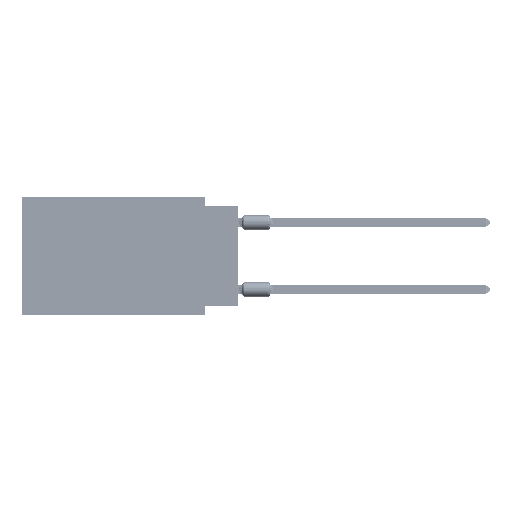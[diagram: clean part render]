
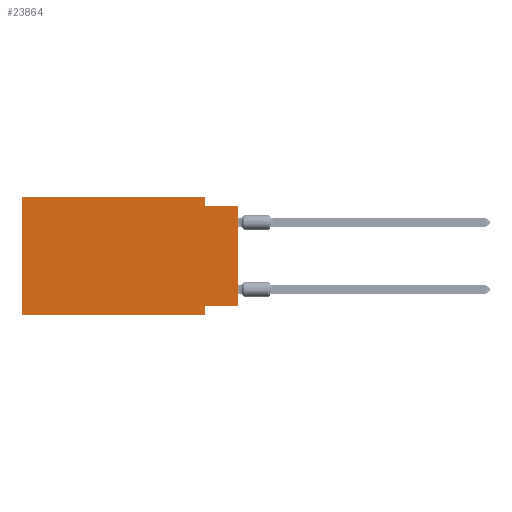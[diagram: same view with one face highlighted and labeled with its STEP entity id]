
A CAD part, left-side view. The second image highlights one B-rep face of the part: STEP entity #23864.
In plain terms, the highlighted planar face has unit normal (-1, 0, 0).
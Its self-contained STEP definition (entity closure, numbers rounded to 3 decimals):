
#1784 = DIRECTION ( 'NONE',  ( 0., -1., 0. ) ) ;
#3954 = ORIENTED_EDGE ( 'NONE', *, *, #64377, .T. ) ;
#4274 = EDGE_CURVE ( 'NONE', #51463, #29022, #56567, .T. ) ;
#5996 = CARTESIAN_POINT ( 'NONE',  ( 0., 2.54, 0. ) ) ;
#6498 = VERTEX_POINT ( 'NONE', #27731 ) ;
#7110 = CARTESIAN_POINT ( 'NONE',  ( 0., 16.383, 0. ) ) ;
#8645 = LINE ( 'NONE', #40354, #41786 ) ;
#8923 = CARTESIAN_POINT ( 'NONE',  ( 0., 0., -0.635 ) ) ;
#9326 = ORIENTED_EDGE ( 'NONE', *, *, #33145, .F. ) ;
#9361 = CARTESIAN_POINT ( 'NONE',  ( 0., 16.383, -8.89 ) ) ;
#11663 = ORIENTED_EDGE ( 'NONE', *, *, #61081, .F. ) ;
#13137 = DIRECTION ( 'NONE',  ( 0., 0., -1. ) ) ;
#14326 = DIRECTION ( 'NONE',  ( 0., 0., -1. ) ) ;
#15035 = DIRECTION ( 'NONE',  ( 0., -1., 0. ) ) ;
#16215 = EDGE_CURVE ( 'NONE', #34249, #54999, #58477, .T. ) ;
#17212 = VERTEX_POINT ( 'NONE', #51149 ) ;
#18328 = DIRECTION ( 'NONE',  ( 0., 0., -1. ) ) ;
#18995 = LINE ( 'NONE', #35566, #62263 ) ;
#19801 = DIRECTION ( 'NONE',  ( 0., 0., 1. ) ) ;
#22435 = CARTESIAN_POINT ( 'NONE',  ( 0., 2.54, -0.635 ) ) ;
#22471 = EDGE_LOOP ( 'NONE', ( #30737, #26094, #35533, #25696, #65704, #3954, #9326, #11663 ) ) ;
#22800 = VECTOR ( 'NONE', #19801, 1000. ) ;
#23864 = ADVANCED_FACE ( 'NONE', ( #63270 ), #43198, .F. ) ;
#24582 = EDGE_CURVE ( 'NONE', #6498, #34249, #60778, .T. ) ;
#25696 = ORIENTED_EDGE ( 'NONE', *, *, #16215, .F. ) ;
#26094 = ORIENTED_EDGE ( 'NONE', *, *, #4274, .F. ) ;
#27631 = VECTOR ( 'NONE', #57805, 1000. ) ;
#27731 = CARTESIAN_POINT ( 'NONE',  ( 0., 16.383, -8.89 ) ) ;
#29022 = VERTEX_POINT ( 'NONE', #8923 ) ;
#30737 = ORIENTED_EDGE ( 'NONE', *, *, #37418, .T. ) ;
#33145 = EDGE_CURVE ( 'NONE', #17212, #58253, #8645, .T. ) ;
#34249 = VERTEX_POINT ( 'NONE', #53157 ) ;
#35364 = CARTESIAN_POINT ( 'NONE',  ( 0., 16.383, 0. ) ) ;
#35533 = ORIENTED_EDGE ( 'NONE', *, *, #36942, .F. ) ;
#35566 = CARTESIAN_POINT ( 'NONE',  ( 0., 2.54, 0. ) ) ;
#35893 = LINE ( 'NONE', #41252, #57654 ) ;
#36942 = EDGE_CURVE ( 'NONE', #54999, #51463, #18995, .T. ) ;
#37418 = EDGE_CURVE ( 'NONE', #56685, #29022, #50862, .T. ) ;
#38509 = DIRECTION ( 'NONE',  ( 1., 0., 0. ) ) ;
#38719 = VECTOR ( 'NONE', #15035, 1000. ) ;
#39641 = CARTESIAN_POINT ( 'NONE',  ( 0., 0., -8.255 ) ) ;
#39847 = CARTESIAN_POINT ( 'NONE',  ( 0., 0., 0. ) ) ;
#40354 = CARTESIAN_POINT ( 'NONE',  ( 0., 2.54, -8.89 ) ) ;
#41252 = CARTESIAN_POINT ( 'NONE',  ( 0., 0., -8.255 ) ) ;
#41786 = VECTOR ( 'NONE', #14326, 1000. ) ;
#42237 = VECTOR ( 'NONE', #61437, 1000. ) ;
#43198 = PLANE ( 'NONE',  #61412 ) ;
#43753 = CARTESIAN_POINT ( 'NONE',  ( 0., 16.383, 0. ) ) ;
#44997 = CARTESIAN_POINT ( 'NONE',  ( 0., 2.54, -8.89 ) ) ;
#45594 = DIRECTION ( 'NONE',  ( 0., 1., 0. ) ) ;
#47536 = CARTESIAN_POINT ( 'NONE',  ( 0., 0., -0.635 ) ) ;
#50773 = LINE ( 'NONE', #9361, #38719 ) ;
#50862 = LINE ( 'NONE', #39847, #22800 ) ;
#51149 = CARTESIAN_POINT ( 'NONE',  ( 0., 2.54, -8.255 ) ) ;
#51463 = VERTEX_POINT ( 'NONE', #22435 ) ;
#53157 = CARTESIAN_POINT ( 'NONE',  ( 0., 16.383, 0. ) ) ;
#54999 = VERTEX_POINT ( 'NONE', #5996 ) ;
#56567 = LINE ( 'NONE', #47536, #57001 ) ;
#56685 = VERTEX_POINT ( 'NONE', #39641 ) ;
#57001 = VECTOR ( 'NONE', #1784, 1000. ) ;
#57654 = VECTOR ( 'NONE', #45594, 1000. ) ;
#57805 = DIRECTION ( 'NONE',  ( 0., -1., 0. ) ) ;
#58253 = VERTEX_POINT ( 'NONE', #44997 ) ;
#58477 = LINE ( 'NONE', #43753, #27631 ) ;
#60778 = LINE ( 'NONE', #35364, #42237 ) ;
#61081 = EDGE_CURVE ( 'NONE', #56685, #17212, #35893, .T. ) ;
#61412 = AXIS2_PLACEMENT_3D ( 'NONE', #7110, #38509, #13137 ) ;
#61437 = DIRECTION ( 'NONE',  ( 0., 0., 1. ) ) ;
#62263 = VECTOR ( 'NONE', #18328, 1000. ) ;
#63270 = FACE_OUTER_BOUND ( 'NONE', #22471, .T. ) ;
#64377 = EDGE_CURVE ( 'NONE', #6498, #58253, #50773, .T. ) ;
#65704 = ORIENTED_EDGE ( 'NONE', *, *, #24582, .F. ) ;
